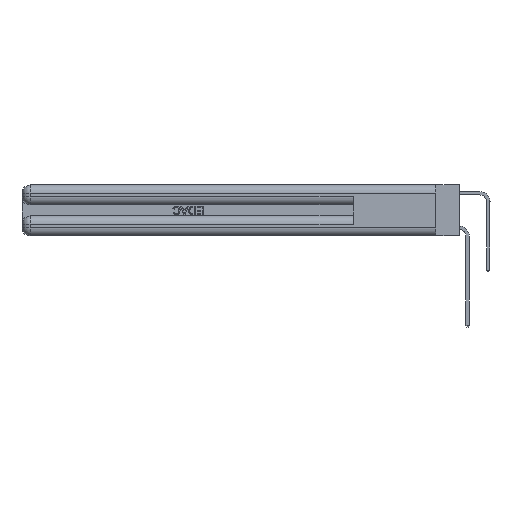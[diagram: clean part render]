
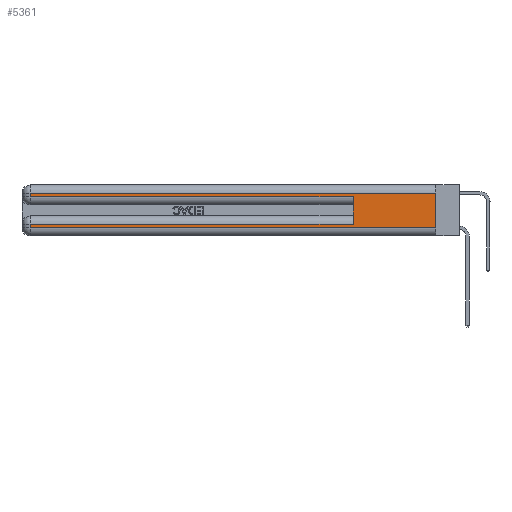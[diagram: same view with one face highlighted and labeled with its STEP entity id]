
A CAD part, left-side view. The second image highlights one B-rep face of the part: STEP entity #5361.
In plain terms, the highlighted planar face has unit normal (-1, 0, 0).
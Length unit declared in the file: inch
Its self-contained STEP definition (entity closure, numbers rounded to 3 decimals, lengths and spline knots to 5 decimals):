
#624 = VECTOR ( 'NONE', #29866, 39.37008 ) ;
#866 = ORIENTED_EDGE ( 'NONE', *, *, #24435, .F. ) ;
#1148 = CARTESIAN_POINT ( 'NONE',  ( 0., 0., 0.06 ) ) ;
#1513 = VERTEX_POINT ( 'NONE', #19775 ) ;
#2375 = ORIENTED_EDGE ( 'NONE', *, *, #5835, .T. ) ;
#2544 = VERTEX_POINT ( 'NONE', #1148 ) ;
#2773 = VERTEX_POINT ( 'NONE', #23134 ) ;
#3060 = EDGE_CURVE ( 'NONE', #6643, #13430, #6290, .T. ) ;
#3166 = LINE ( 'NONE', #21588, #8000 ) ;
#3315 = LINE ( 'NONE', #29676, #31218 ) ;
#3467 = FACE_OUTER_BOUND ( 'NONE', #8259, .T. ) ;
#3639 = CARTESIAN_POINT ( 'NONE',  ( 0., 0., 0.085 ) ) ;
#4419 = LINE ( 'NONE', #7175, #14071 ) ;
#4758 = VECTOR ( 'NONE', #32023, 39.37008 ) ;
#5257 = VERTEX_POINT ( 'NONE', #27501 ) ;
#5361 = ADVANCED_FACE ( 'NONE', ( #3467 ), #7441, .F. ) ;
#5835 = EDGE_CURVE ( 'NONE', #35896, #2544, #27010, .T. ) ;
#6290 = LINE ( 'NONE', #3639, #19322 ) ;
#6398 = DIRECTION ( 'NONE',  ( 0., 0., -1. ) ) ;
#6643 = VERTEX_POINT ( 'NONE', #10445 ) ;
#7082 = ORIENTED_EDGE ( 'NONE', *, *, #19287, .T. ) ;
#7175 = CARTESIAN_POINT ( 'NONE',  ( 0., 0., 0.37 ) ) ;
#7441 = PLANE ( 'NONE',  #30861 ) ;
#8000 = VECTOR ( 'NONE', #35370, 39.37008 ) ;
#8109 = LINE ( 'NONE', #30107, #624 ) ;
#8259 = EDGE_LOOP ( 'NONE', ( #13494, #7082, #30985, #13412, #866, #14568, #26441, #2375 ) ) ;
#8999 = CARTESIAN_POINT ( 'NONE',  ( 0., 0., 0.31 ) ) ;
#9517 = CARTESIAN_POINT ( 'NONE',  ( 0., 0., 0.06 ) ) ;
#9893 = DIRECTION ( 'NONE',  ( 1., 0., 0. ) ) ;
#10445 = CARTESIAN_POINT ( 'NONE',  ( 0., 0.6, 0.085 ) ) ;
#10697 = VECTOR ( 'NONE', #34652, 39.37008 ) ;
#10884 = VECTOR ( 'NONE', #6398, 39.37008 ) ;
#12971 = CARTESIAN_POINT ( 'NONE',  ( 0., 0.6, 0.285 ) ) ;
#13412 = ORIENTED_EDGE ( 'NONE', *, *, #22892, .T. ) ;
#13430 = VERTEX_POINT ( 'NONE', #35177 ) ;
#13494 = ORIENTED_EDGE ( 'NONE', *, *, #27829, .F. ) ;
#14071 = VECTOR ( 'NONE', #26648, 39.37008 ) ;
#14385 = LINE ( 'NONE', #20498, #10884 ) ;
#14443 = VERTEX_POINT ( 'NONE', #12971 ) ;
#14568 = ORIENTED_EDGE ( 'NONE', *, *, #3060, .T. ) ;
#19287 = EDGE_CURVE ( 'NONE', #1513, #5257, #20710, .T. ) ;
#19322 = VECTOR ( 'NONE', #19836, 39.37008 ) ;
#19731 = EDGE_CURVE ( 'NONE', #5257, #2773, #14385, .T. ) ;
#19775 = CARTESIAN_POINT ( 'NONE',  ( 0., 0., 0.31 ) ) ;
#19836 = DIRECTION ( 'NONE',  ( 0., 1., 0. ) ) ;
#20498 = CARTESIAN_POINT ( 'NONE',  ( 0., 2.94, 0.37 ) ) ;
#20710 = LINE ( 'NONE', #8999, #10697 ) ;
#21588 = CARTESIAN_POINT ( 'NONE',  ( 0., 0.6, 0.145 ) ) ;
#22892 = EDGE_CURVE ( 'NONE', #2773, #14443, #8109, .T. ) ;
#23134 = CARTESIAN_POINT ( 'NONE',  ( 0., 2.94, 0.285 ) ) ;
#23978 = CARTESIAN_POINT ( 'NONE',  ( 0., 0., 0.37 ) ) ;
#24215 = CARTESIAN_POINT ( 'NONE',  ( 0., 2.94, 0.06 ) ) ;
#24435 = EDGE_CURVE ( 'NONE', #6643, #14443, #3166, .T. ) ;
#26441 = ORIENTED_EDGE ( 'NONE', *, *, #33425, .T. ) ;
#26648 = DIRECTION ( 'NONE',  ( 0., 0., -1. ) ) ;
#27010 = LINE ( 'NONE', #9517, #4758 ) ;
#27501 = CARTESIAN_POINT ( 'NONE',  ( 0., 2.94, 0.31 ) ) ;
#27829 = EDGE_CURVE ( 'NONE', #1513, #2544, #4419, .T. ) ;
#29348 = DIRECTION ( 'NONE',  ( 0., 0., -1. ) ) ;
#29676 = CARTESIAN_POINT ( 'NONE',  ( 0., 2.94, 0.37 ) ) ;
#29866 = DIRECTION ( 'NONE',  ( 0., -1., 0. ) ) ;
#29906 = DIRECTION ( 'NONE',  ( 0., 0., -1. ) ) ;
#30107 = CARTESIAN_POINT ( 'NONE',  ( 0., 0., 0.285 ) ) ;
#30861 = AXIS2_PLACEMENT_3D ( 'NONE', #23978, #9893, #29348 ) ;
#30985 = ORIENTED_EDGE ( 'NONE', *, *, #19731, .T. ) ;
#31218 = VECTOR ( 'NONE', #29906, 39.37008 ) ;
#32023 = DIRECTION ( 'NONE',  ( 0., -1., 0. ) ) ;
#33425 = EDGE_CURVE ( 'NONE', #13430, #35896, #3315, .T. ) ;
#34652 = DIRECTION ( 'NONE',  ( 0., 1., 0. ) ) ;
#35177 = CARTESIAN_POINT ( 'NONE',  ( 0., 2.94, 0.085 ) ) ;
#35370 = DIRECTION ( 'NONE',  ( 0., 0., 1. ) ) ;
#35896 = VERTEX_POINT ( 'NONE', #24215 ) ;
